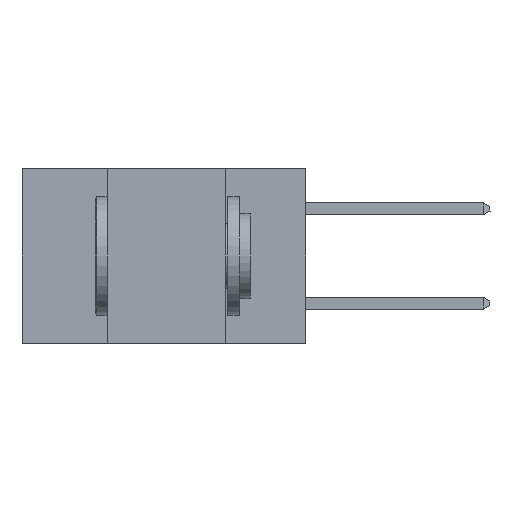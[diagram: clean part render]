
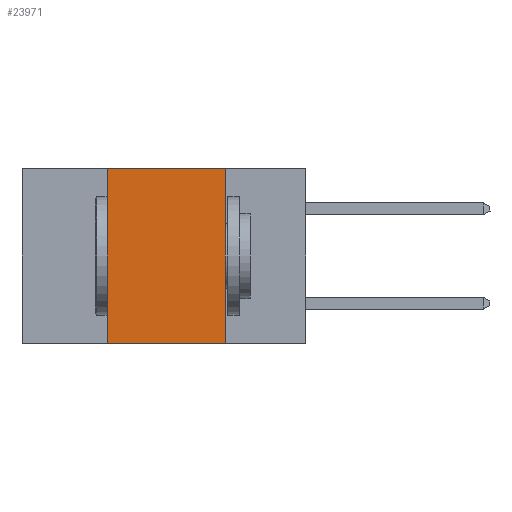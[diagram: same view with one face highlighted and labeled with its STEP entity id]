
A CAD part, left-side view. The second image highlights one B-rep face of the part: STEP entity #23971.
In plain terms, the highlighted planar face has unit normal (-1, 0, 0).
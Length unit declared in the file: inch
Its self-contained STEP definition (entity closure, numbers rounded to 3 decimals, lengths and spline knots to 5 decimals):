
#263 = CARTESIAN_POINT ( 'NONE',  ( 0., 0.17, 0. ) ) ;
#686 = ORIENTED_EDGE ( 'NONE', *, *, #4341, .F. ) ;
#1125 = ORIENTED_EDGE ( 'NONE', *, *, #24147, .F. ) ;
#1535 = DIRECTION ( 'NONE',  ( 0., 0., -1. ) ) ;
#1683 = DIRECTION ( 'NONE',  ( 0., -1., 0. ) ) ;
#3001 = CARTESIAN_POINT ( 'NONE',  ( 0., 0.17, -0.37 ) ) ;
#3782 = EDGE_LOOP ( 'NONE', ( #14699, #686, #1125, #10108 ) ) ;
#4341 = EDGE_CURVE ( 'NONE', #6220, #12135, #12972, .T. ) ;
#4659 = FACE_OUTER_BOUND ( 'NONE', #3782, .T. ) ;
#4685 = CARTESIAN_POINT ( 'NONE',  ( 0., 0.42, 0. ) ) ;
#5165 = EDGE_CURVE ( 'NONE', #12135, #7899, #24178, .T. ) ;
#6220 = VERTEX_POINT ( 'NONE', #4685 ) ;
#7899 = VERTEX_POINT ( 'NONE', #3001 ) ;
#8830 = CARTESIAN_POINT ( 'NONE',  ( 0., 0.42, -0.37 ) ) ;
#10108 = ORIENTED_EDGE ( 'NONE', *, *, #11836, .T. ) ;
#10908 = LINE ( 'NONE', #25318, #15433 ) ;
#11836 = EDGE_CURVE ( 'NONE', #16558, #7899, #10908, .T. ) ;
#12135 = VERTEX_POINT ( 'NONE', #22230 ) ;
#12927 = CARTESIAN_POINT ( 'NONE',  ( 0., 0.6, 0. ) ) ;
#12972 = LINE ( 'NONE', #12927, #17570 ) ;
#13561 = DIRECTION ( 'NONE',  ( 1., 0., 0. ) ) ;
#13833 = VECTOR ( 'NONE', #15874, 39.37008 ) ;
#14699 = ORIENTED_EDGE ( 'NONE', *, *, #5165, .F. ) ;
#15433 = VECTOR ( 'NONE', #1683, 39.37008 ) ;
#15874 = DIRECTION ( 'NONE',  ( 0., 0., -1. ) ) ;
#15881 = VECTOR ( 'NONE', #24832, 39.37008 ) ;
#16558 = VERTEX_POINT ( 'NONE', #8830 ) ;
#17570 = VECTOR ( 'NONE', #21884, 39.37008 ) ;
#19304 = CARTESIAN_POINT ( 'NONE',  ( 0., 0.6, 0. ) ) ;
#20998 = CARTESIAN_POINT ( 'NONE',  ( 0., 0.42, 0. ) ) ;
#21093 = LINE ( 'NONE', #20998, #15881 ) ;
#21493 = AXIS2_PLACEMENT_3D ( 'NONE', #19304, #13561, #1535 ) ;
#21884 = DIRECTION ( 'NONE',  ( 0., -1., 0. ) ) ;
#22230 = CARTESIAN_POINT ( 'NONE',  ( 0., 0.17, 0. ) ) ;
#23971 = ADVANCED_FACE ( 'NONE', ( #4659 ), #25175, .F. ) ;
#24147 = EDGE_CURVE ( 'NONE', #16558, #6220, #21093, .T. ) ;
#24178 = LINE ( 'NONE', #263, #13833 ) ;
#24832 = DIRECTION ( 'NONE',  ( 0., 0., 1. ) ) ;
#25175 = PLANE ( 'NONE',  #21493 ) ;
#25318 = CARTESIAN_POINT ( 'NONE',  ( 0., 0.6, -0.37 ) ) ;
